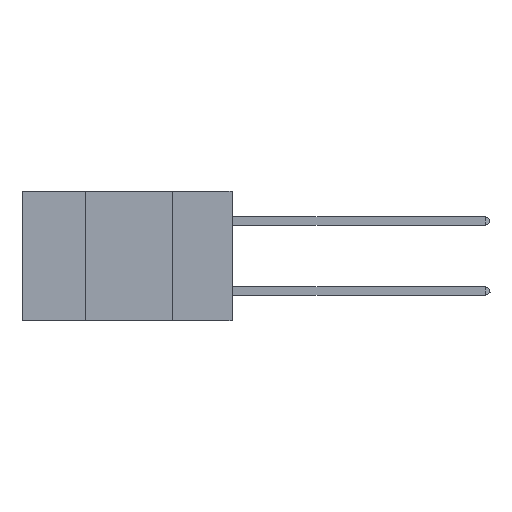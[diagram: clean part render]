
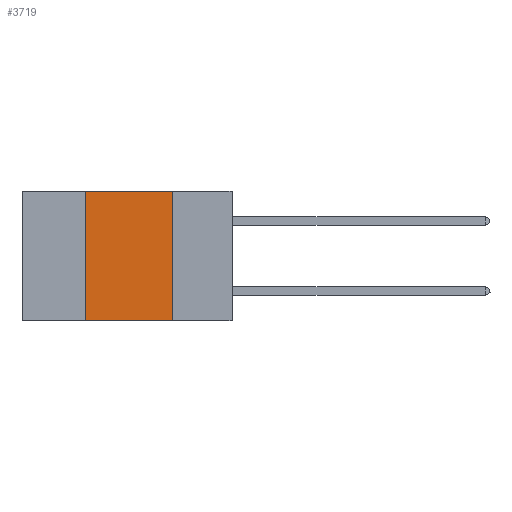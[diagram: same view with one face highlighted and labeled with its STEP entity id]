
A CAD part, left-side view. The second image highlights one B-rep face of the part: STEP entity #3719.
In plain terms, the highlighted planar face has unit normal (-1, 0, 0).
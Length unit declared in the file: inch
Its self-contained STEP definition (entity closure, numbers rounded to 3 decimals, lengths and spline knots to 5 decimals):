
#470 = CARTESIAN_POINT ( 'NONE',  ( 0., 0.6, 0. ) ) ;
#568 = DIRECTION ( 'NONE',  ( 0., 0., -1. ) ) ;
#1645 = EDGE_CURVE ( 'NONE', #3450, #4975, #12861, .T. ) ;
#1894 = CARTESIAN_POINT ( 'NONE',  ( 0., 0.17, 0. ) ) ;
#3030 = DIRECTION ( 'NONE',  ( 0., 0., -1. ) ) ;
#3070 = LINE ( 'NONE', #8973, #12637 ) ;
#3135 = ORIENTED_EDGE ( 'NONE', *, *, #9292, .F. ) ;
#3189 = EDGE_CURVE ( 'NONE', #3450, #6288, #10383, .T. ) ;
#3450 = VERTEX_POINT ( 'NONE', #7674 ) ;
#3480 = CARTESIAN_POINT ( 'NONE',  ( 0., 0.42, 0. ) ) ;
#3719 = ADVANCED_FACE ( 'NONE', ( #12977 ), #8137, .F. ) ;
#4409 = DIRECTION ( 'NONE',  ( 0., -1., 0. ) ) ;
#4919 = VECTOR ( 'NONE', #4409, 39.37008 ) ;
#4975 = VERTEX_POINT ( 'NONE', #3480 ) ;
#5257 = VECTOR ( 'NONE', #5283, 39.37008 ) ;
#5283 = DIRECTION ( 'NONE',  ( 0., -1., 0. ) ) ;
#5496 = CARTESIAN_POINT ( 'NONE',  ( 0., 0.6, -0.37 ) ) ;
#5785 = CARTESIAN_POINT ( 'NONE',  ( 0., 0.42, 0. ) ) ;
#5793 = AXIS2_PLACEMENT_3D ( 'NONE', #470, #6587, #568 ) ;
#6288 = VERTEX_POINT ( 'NONE', #8274 ) ;
#6392 = EDGE_LOOP ( 'NONE', ( #11117, #3135, #6540, #11781 ) ) ;
#6540 = ORIENTED_EDGE ( 'NONE', *, *, #1645, .F. ) ;
#6587 = DIRECTION ( 'NONE',  ( 1., 0., 0. ) ) ;
#7087 = EDGE_CURVE ( 'NONE', #13415, #6288, #3070, .T. ) ;
#7674 = CARTESIAN_POINT ( 'NONE',  ( 0., 0.42, -0.37 ) ) ;
#8137 = PLANE ( 'NONE',  #5793 ) ;
#8274 = CARTESIAN_POINT ( 'NONE',  ( 0., 0.17, -0.37 ) ) ;
#8336 = VECTOR ( 'NONE', #15508, 39.37008 ) ;
#8973 = CARTESIAN_POINT ( 'NONE',  ( 0., 0.17, 0. ) ) ;
#9292 = EDGE_CURVE ( 'NONE', #4975, #13415, #14091, .T. ) ;
#10383 = LINE ( 'NONE', #5496, #4919 ) ;
#11117 = ORIENTED_EDGE ( 'NONE', *, *, #7087, .F. ) ;
#11781 = ORIENTED_EDGE ( 'NONE', *, *, #3189, .T. ) ;
#12472 = CARTESIAN_POINT ( 'NONE',  ( 0., 0.6, 0. ) ) ;
#12637 = VECTOR ( 'NONE', #3030, 39.37008 ) ;
#12861 = LINE ( 'NONE', #5785, #8336 ) ;
#12977 = FACE_OUTER_BOUND ( 'NONE', #6392, .T. ) ;
#13415 = VERTEX_POINT ( 'NONE', #1894 ) ;
#14091 = LINE ( 'NONE', #12472, #5257 ) ;
#15508 = DIRECTION ( 'NONE',  ( 0., 0., 1. ) ) ;
